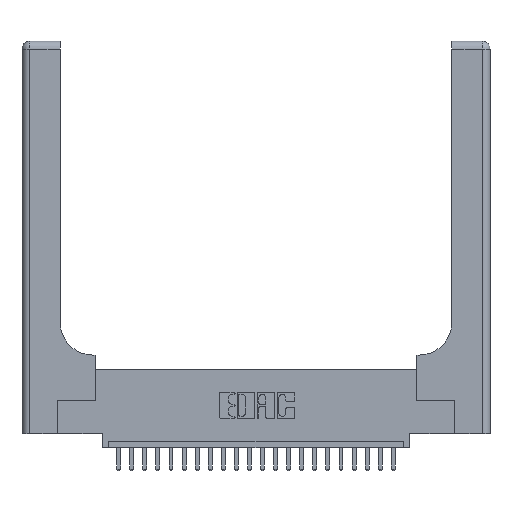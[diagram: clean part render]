
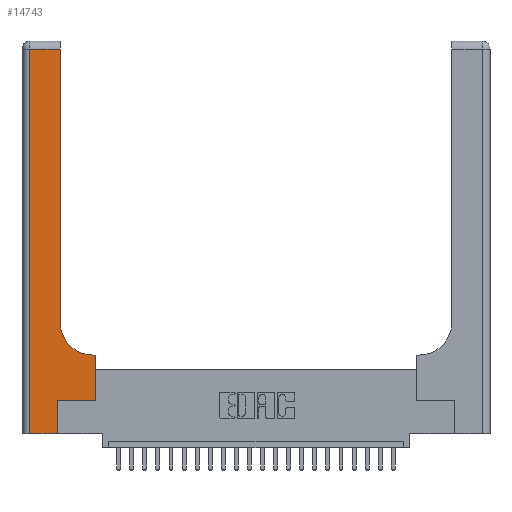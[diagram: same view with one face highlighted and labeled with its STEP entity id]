
A CAD part, top view. The second image highlights one B-rep face of the part: STEP entity #14743.
In plain terms, the highlighted planar face has unit normal (0, 0, 1).
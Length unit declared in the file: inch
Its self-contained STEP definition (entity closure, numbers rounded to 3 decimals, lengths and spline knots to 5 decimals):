
#14 = LINE ( 'NONE', #8657, #19689 ) ;
#143 = ORIENTED_EDGE ( 'NONE', *, *, #10658, .T. ) ;
#231 = CARTESIAN_POINT ( 'NONE',  ( 0.2915, 3., 0.37 ) ) ;
#792 = CARTESIAN_POINT ( 'NONE',  ( 0.5585, 0.25, 0.37 ) ) ;
#808 = FACE_OUTER_BOUND ( 'NONE', #9970, .T. ) ;
#820 = VECTOR ( 'NONE', #23339, 39.37008 ) ;
#1086 = LINE ( 'NONE', #18982, #16871 ) ;
#1239 = DIRECTION ( 'NONE',  ( 0., 1., 0. ) ) ;
#1672 = EDGE_CURVE ( 'NONE', #21811, #16022, #20720, .T. ) ;
#2065 = ORIENTED_EDGE ( 'NONE', *, *, #12001, .T. ) ;
#2067 = DIRECTION ( 'NONE',  ( 0., 1., 0. ) ) ;
#3083 = CARTESIAN_POINT ( 'NONE',  ( 0.06, 0., 0.37 ) ) ;
#3586 = CARTESIAN_POINT ( 'NONE',  ( 0.269, 0.25, 0.37 ) ) ;
#3788 = CARTESIAN_POINT ( 'NONE',  ( 0.2915, 0.85, 0.37 ) ) ;
#4146 = VERTEX_POINT ( 'NONE', #6634 ) ;
#4195 = VECTOR ( 'NONE', #9742, 39.37008 ) ;
#5032 = VERTEX_POINT ( 'NONE', #24507 ) ;
#5222 = DIRECTION ( 'NONE',  ( 1., 0., 0. ) ) ;
#5284 = LINE ( 'NONE', #14097, #820 ) ;
#5990 = DIRECTION ( 'NONE',  ( 1., 0., 0. ) ) ;
#6092 = ORIENTED_EDGE ( 'NONE', *, *, #11145, .T. ) ;
#6157 = VECTOR ( 'NONE', #1239, 39.37008 ) ;
#6187 = ORIENTED_EDGE ( 'NONE', *, *, #1672, .T. ) ;
#6444 = LINE ( 'NONE', #20237, #6157 ) ;
#6622 = EDGE_CURVE ( 'NONE', #22414, #5032, #5284, .T. ) ;
#6634 = CARTESIAN_POINT ( 'NONE',  ( 0.06, 2.94, 0.37 ) ) ;
#6645 = DIRECTION ( 'NONE',  ( -1., 0., 0. ) ) ;
#7174 = EDGE_CURVE ( 'NONE', #19013, #11346, #1086, .T. ) ;
#7492 = VECTOR ( 'NONE', #2067, 39.37008 ) ;
#8657 = CARTESIAN_POINT ( 'NONE',  ( 0., 2.94, 0.37 ) ) ;
#9742 = DIRECTION ( 'NONE',  ( 0., 1., 0. ) ) ;
#9970 = EDGE_LOOP ( 'NONE', ( #18958, #2065, #143, #24013, #6092, #24599, #12590, #24700, #6187 ) ) ;
#10475 = AXIS2_PLACEMENT_3D ( 'NONE', #24476, #16811, #5222 ) ;
#10595 = VERTEX_POINT ( 'NONE', #19883 ) ;
#10658 = EDGE_CURVE ( 'NONE', #4146, #22414, #22144, .T. ) ;
#11112 = PLANE ( 'NONE',  #19294 ) ;
#11145 = EDGE_CURVE ( 'NONE', #5032, #19013, #21812, .T. ) ;
#11346 = VERTEX_POINT ( 'NONE', #792 ) ;
#12001 = EDGE_CURVE ( 'NONE', #10595, #4146, #14, .T. ) ;
#12410 = EDGE_CURVE ( 'NONE', #16022, #10595, #12559, .T. ) ;
#12559 = LINE ( 'NONE', #231, #4195 ) ;
#12590 = ORIENTED_EDGE ( 'NONE', *, *, #15310, .T. ) ;
#13015 = CARTESIAN_POINT ( 'NONE',  ( 0., 3., 0.37 ) ) ;
#13223 = LINE ( 'NONE', #19902, #22740 ) ;
#14097 = CARTESIAN_POINT ( 'NONE',  ( 0., 0., 0.37 ) ) ;
#14683 = VECTOR ( 'NONE', #19706, 39.37008 ) ;
#14743 = ADVANCED_FACE ( 'NONE', ( #808 ), #11112, .F. ) ;
#15294 = CARTESIAN_POINT ( 'NONE',  ( 0.269, 0., 0.37 ) ) ;
#15305 = VERTEX_POINT ( 'NONE', #22379 ) ;
#15310 = EDGE_CURVE ( 'NONE', #11346, #15305, #6444, .T. ) ;
#15333 = DIRECTION ( 'NONE',  ( 0., 0., -1. ) ) ;
#15883 = CARTESIAN_POINT ( 'NONE',  ( 0.06, 3., 0.37 ) ) ;
#16022 = VERTEX_POINT ( 'NONE', #3788 ) ;
#16504 = CARTESIAN_POINT ( 'NONE',  ( 0.5415, 0.6, 0.37 ) ) ;
#16811 = DIRECTION ( 'NONE',  ( 0., 0., -1. ) ) ;
#16871 = VECTOR ( 'NONE', #5990, 39.37008 ) ;
#17515 = EDGE_CURVE ( 'NONE', #15305, #21811, #13223, .T. ) ;
#18958 = ORIENTED_EDGE ( 'NONE', *, *, #12410, .T. ) ;
#18982 = CARTESIAN_POINT ( 'NONE',  ( 0.269, 0.25, 0.37 ) ) ;
#19013 = VERTEX_POINT ( 'NONE', #3586 ) ;
#19248 = DIRECTION ( 'NONE',  ( -1., 0., 0. ) ) ;
#19294 = AXIS2_PLACEMENT_3D ( 'NONE', #13015, #15333, #19248 ) ;
#19689 = VECTOR ( 'NONE', #21999, 39.37008 ) ;
#19706 = DIRECTION ( 'NONE',  ( 0., -1., 0. ) ) ;
#19883 = CARTESIAN_POINT ( 'NONE',  ( 0.2915, 2.94, 0.37 ) ) ;
#19902 = CARTESIAN_POINT ( 'NONE',  ( 0.2915, 0.6, 0.37 ) ) ;
#20237 = CARTESIAN_POINT ( 'NONE',  ( 0.5585, 0.25, 0.37 ) ) ;
#20720 = CIRCLE ( 'NONE', #10475, 0.25 ) ;
#21811 = VERTEX_POINT ( 'NONE', #16504 ) ;
#21812 = LINE ( 'NONE', #15294, #7492 ) ;
#21999 = DIRECTION ( 'NONE',  ( -1., 0., 0. ) ) ;
#22144 = LINE ( 'NONE', #15883, #14683 ) ;
#22379 = CARTESIAN_POINT ( 'NONE',  ( 0.5585, 0.6, 0.37 ) ) ;
#22414 = VERTEX_POINT ( 'NONE', #3083 ) ;
#22740 = VECTOR ( 'NONE', #6645, 39.37008 ) ;
#23339 = DIRECTION ( 'NONE',  ( 1., 0., 0. ) ) ;
#24013 = ORIENTED_EDGE ( 'NONE', *, *, #6622, .T. ) ;
#24476 = CARTESIAN_POINT ( 'NONE',  ( 0.5415, 0.85, 0.37 ) ) ;
#24507 = CARTESIAN_POINT ( 'NONE',  ( 0.269, 0., 0.37 ) ) ;
#24599 = ORIENTED_EDGE ( 'NONE', *, *, #7174, .T. ) ;
#24700 = ORIENTED_EDGE ( 'NONE', *, *, #17515, .T. ) ;
